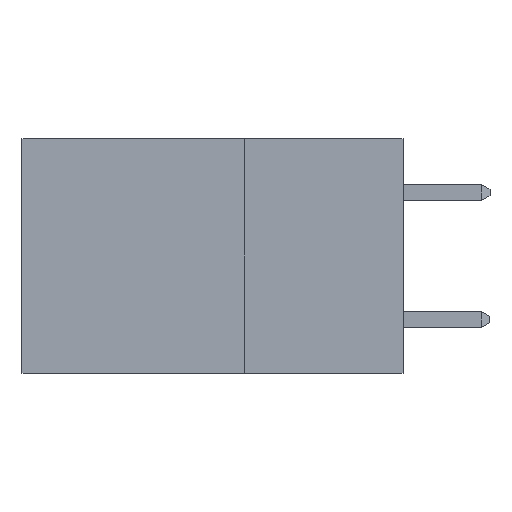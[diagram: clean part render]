
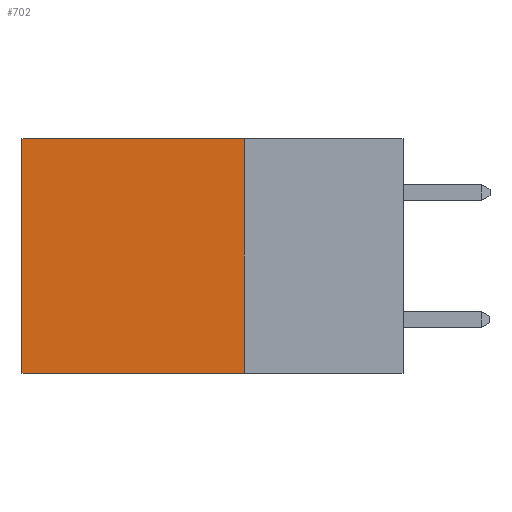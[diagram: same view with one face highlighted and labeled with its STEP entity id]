
A CAD part, left-side view. The second image highlights one B-rep face of the part: STEP entity #702.
In plain terms, the highlighted planar face has unit normal (-1, 0, 0).
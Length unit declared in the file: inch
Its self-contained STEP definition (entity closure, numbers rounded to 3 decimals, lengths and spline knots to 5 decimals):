
#409 = EDGE_CURVE ( 'NONE', #7305, #2126, #7194, .T. ) ;
#681 = VECTOR ( 'NONE', #7799, 39.37008 ) ;
#686 = CARTESIAN_POINT ( 'NONE',  ( 0.2875, 0.25, 0. ) ) ;
#702 = ADVANCED_FACE ( 'NONE', ( #9045 ), #1493, .F. ) ;
#869 = ORIENTED_EDGE ( 'NONE', *, *, #409, .T. ) ;
#1190 = VERTEX_POINT ( 'NONE', #6856 ) ;
#1493 = PLANE ( 'NONE',  #7846 ) ;
#1870 = EDGE_CURVE ( 'NONE', #2126, #7263, #2820, .T. ) ;
#2126 = VERTEX_POINT ( 'NONE', #3918 ) ;
#2507 = ORIENTED_EDGE ( 'NONE', *, *, #4555, .F. ) ;
#2820 = LINE ( 'NONE', #9151, #6893 ) ;
#3256 = VECTOR ( 'NONE', #3957, 39.37008 ) ;
#3775 = DIRECTION ( 'NONE',  ( 0., 0., -1. ) ) ;
#3785 = DIRECTION ( 'NONE',  ( 0., 0., -1. ) ) ;
#3918 = CARTESIAN_POINT ( 'NONE',  ( 0.2875, 0.6, 0. ) ) ;
#3957 = DIRECTION ( 'NONE',  ( 0., 1., 0. ) ) ;
#4188 = DIRECTION ( 'NONE',  ( 0., 1., 0. ) ) ;
#4232 = EDGE_CURVE ( 'NONE', #7305, #1190, #6876, .T. ) ;
#4555 = EDGE_CURVE ( 'NONE', #1190, #7263, #5904, .T. ) ;
#5196 = DIRECTION ( 'NONE',  ( 1., 0., 0. ) ) ;
#5563 = EDGE_LOOP ( 'NONE', ( #6323, #2507, #9367, #869 ) ) ;
#5867 = CARTESIAN_POINT ( 'NONE',  ( 0.2875, 0.6, -0.37 ) ) ;
#5904 = LINE ( 'NONE', #6666, #7488 ) ;
#6229 = CARTESIAN_POINT ( 'NONE',  ( 0.2875, 0.25, 0. ) ) ;
#6323 = ORIENTED_EDGE ( 'NONE', *, *, #1870, .T. ) ;
#6666 = CARTESIAN_POINT ( 'NONE',  ( 0.2875, 0.25, -0.37 ) ) ;
#6856 = CARTESIAN_POINT ( 'NONE',  ( 0.2875, 0.25, -0.37 ) ) ;
#6876 = LINE ( 'NONE', #8501, #681 ) ;
#6893 = VECTOR ( 'NONE', #3785, 39.37008 ) ;
#7194 = LINE ( 'NONE', #6229, #3256 ) ;
#7263 = VERTEX_POINT ( 'NONE', #5867 ) ;
#7305 = VERTEX_POINT ( 'NONE', #8106 ) ;
#7488 = VECTOR ( 'NONE', #4188, 39.37008 ) ;
#7799 = DIRECTION ( 'NONE',  ( 0., 0., -1. ) ) ;
#7846 = AXIS2_PLACEMENT_3D ( 'NONE', #686, #5196, #3775 ) ;
#8106 = CARTESIAN_POINT ( 'NONE',  ( 0.2875, 0.25, 0. ) ) ;
#8501 = CARTESIAN_POINT ( 'NONE',  ( 0.2875, 0.25, 0. ) ) ;
#9045 = FACE_OUTER_BOUND ( 'NONE', #5563, .T. ) ;
#9151 = CARTESIAN_POINT ( 'NONE',  ( 0.2875, 0.6, 0. ) ) ;
#9367 = ORIENTED_EDGE ( 'NONE', *, *, #4232, .F. ) ;
